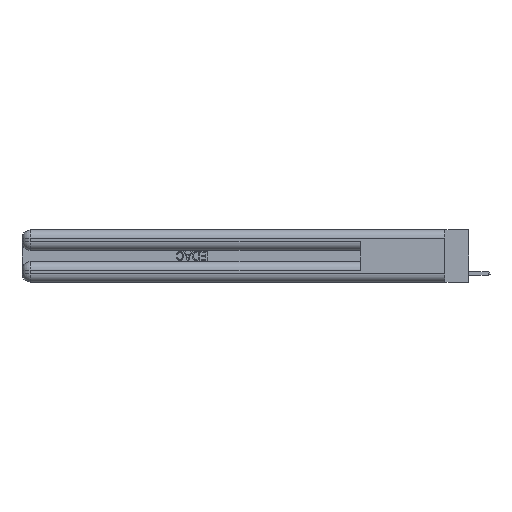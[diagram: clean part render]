
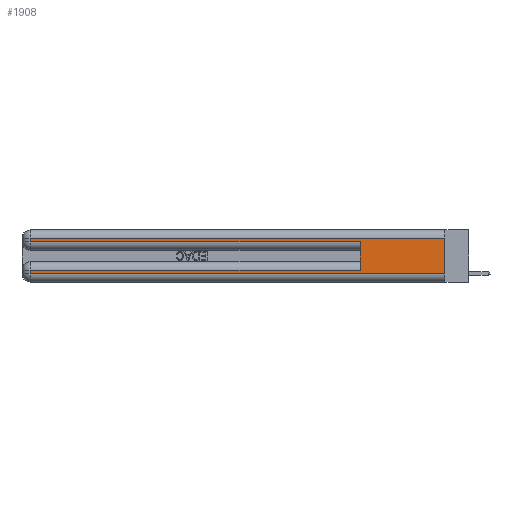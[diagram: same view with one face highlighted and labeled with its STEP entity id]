
A CAD part, left-side view. The second image highlights one B-rep face of the part: STEP entity #1908.
In plain terms, the highlighted planar face has unit normal (-1, 0, 0).
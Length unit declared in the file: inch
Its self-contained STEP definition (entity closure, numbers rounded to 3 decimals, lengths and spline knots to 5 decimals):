
#291 = CARTESIAN_POINT ( 'NONE',  ( 0., 0., 0.37 ) ) ;
#361 = AXIS2_PLACEMENT_3D ( 'NONE', #291, #21021, #10533 ) ;
#381 = CARTESIAN_POINT ( 'NONE',  ( 0., 0.6, 0.085 ) ) ;
#1177 = EDGE_CURVE ( 'NONE', #16755, #10103, #4857, .T. ) ;
#1198 = DIRECTION ( 'NONE',  ( 0., 0., 1. ) ) ;
#1211 = ORIENTED_EDGE ( 'NONE', *, *, #25417, .T. ) ;
#1470 = LINE ( 'NONE', #20380, #2136 ) ;
#1558 = VECTOR ( 'NONE', #1198, 39.37008 ) ;
#1616 = ORIENTED_EDGE ( 'NONE', *, *, #2651, .T. ) ;
#1734 = VECTOR ( 'NONE', #12734, 39.37008 ) ;
#1908 = ADVANCED_FACE ( 'NONE', ( #14744 ), #21427, .F. ) ;
#1928 = VERTEX_POINT ( 'NONE', #25392 ) ;
#2090 = ORIENTED_EDGE ( 'NONE', *, *, #19358, .F. ) ;
#2124 = DIRECTION ( 'NONE',  ( 0., 1., 0. ) ) ;
#2135 = EDGE_CURVE ( 'NONE', #21416, #1928, #24283, .T. ) ;
#2136 = VECTOR ( 'NONE', #7729, 39.37008 ) ;
#2368 = CARTESIAN_POINT ( 'NONE',  ( 0., 2.94, 0.37 ) ) ;
#2477 = VERTEX_POINT ( 'NONE', #16028 ) ;
#2498 = LINE ( 'NONE', #2368, #1734 ) ;
#2587 = VECTOR ( 'NONE', #23390, 39.37008 ) ;
#2651 = EDGE_CURVE ( 'NONE', #9001, #1928, #22695, .T. ) ;
#2717 = ORIENTED_EDGE ( 'NONE', *, *, #9899, .T. ) ;
#3200 = CARTESIAN_POINT ( 'NONE',  ( 0., 0., 0.31 ) ) ;
#3744 = CARTESIAN_POINT ( 'NONE',  ( 0., 0., 0.06 ) ) ;
#4393 = CARTESIAN_POINT ( 'NONE',  ( 0., 2.94, 0.285 ) ) ;
#4735 = EDGE_CURVE ( 'NONE', #26776, #7300, #1470, .T. ) ;
#4857 = LINE ( 'NONE', #15074, #2587 ) ;
#5105 = ORIENTED_EDGE ( 'NONE', *, *, #1177, .T. ) ;
#6921 = VECTOR ( 'NONE', #18528, 39.37008 ) ;
#7300 = VERTEX_POINT ( 'NONE', #13437 ) ;
#7481 = LINE ( 'NONE', #19456, #1558 ) ;
#7729 = DIRECTION ( 'NONE',  ( 0., -1., 0. ) ) ;
#9001 = VERTEX_POINT ( 'NONE', #24707 ) ;
#9186 = VECTOR ( 'NONE', #20363, 39.37008 ) ;
#9899 = EDGE_CURVE ( 'NONE', #21416, #2477, #20532, .T. ) ;
#10103 = VERTEX_POINT ( 'NONE', #21466 ) ;
#10351 = EDGE_LOOP ( 'NONE', ( #10614, #2717, #1211, #20136, #2090, #5105, #12461, #1616 ) ) ;
#10533 = DIRECTION ( 'NONE',  ( 0., 0., -1. ) ) ;
#10614 = ORIENTED_EDGE ( 'NONE', *, *, #2135, .F. ) ;
#11387 = CARTESIAN_POINT ( 'NONE',  ( 0., 2.94, 0.37 ) ) ;
#12461 = ORIENTED_EDGE ( 'NONE', *, *, #12863, .T. ) ;
#12734 = DIRECTION ( 'NONE',  ( 0., 0., -1. ) ) ;
#12863 = EDGE_CURVE ( 'NONE', #10103, #9001, #21742, .T. ) ;
#13144 = VECTOR ( 'NONE', #25565, 39.37008 ) ;
#13437 = CARTESIAN_POINT ( 'NONE',  ( 0., 0.6, 0.285 ) ) ;
#14744 = FACE_OUTER_BOUND ( 'NONE', #10351, .T. ) ;
#15074 = CARTESIAN_POINT ( 'NONE',  ( 0., 0., 0.085 ) ) ;
#16028 = CARTESIAN_POINT ( 'NONE',  ( 0., 2.94, 0.31 ) ) ;
#16755 = VERTEX_POINT ( 'NONE', #381 ) ;
#18528 = DIRECTION ( 'NONE',  ( 0., 0., -1. ) ) ;
#19358 = EDGE_CURVE ( 'NONE', #16755, #7300, #7481, .T. ) ;
#19456 = CARTESIAN_POINT ( 'NONE',  ( 0., 0.6, 0.145 ) ) ;
#20120 = VECTOR ( 'NONE', #2124, 39.37008 ) ;
#20136 = ORIENTED_EDGE ( 'NONE', *, *, #4735, .T. ) ;
#20363 = DIRECTION ( 'NONE',  ( 0., -1., 0. ) ) ;
#20380 = CARTESIAN_POINT ( 'NONE',  ( 0., 0., 0.285 ) ) ;
#20430 = CARTESIAN_POINT ( 'NONE',  ( 0., 0., 0.37 ) ) ;
#20532 = LINE ( 'NONE', #22461, #20120 ) ;
#21021 = DIRECTION ( 'NONE',  ( 1., 0., 0. ) ) ;
#21416 = VERTEX_POINT ( 'NONE', #3200 ) ;
#21427 = PLANE ( 'NONE',  #361 ) ;
#21466 = CARTESIAN_POINT ( 'NONE',  ( 0., 2.94, 0.085 ) ) ;
#21742 = LINE ( 'NONE', #11387, #13144 ) ;
#22461 = CARTESIAN_POINT ( 'NONE',  ( 0., 0., 0.31 ) ) ;
#22695 = LINE ( 'NONE', #3744, #9186 ) ;
#23390 = DIRECTION ( 'NONE',  ( 0., 1., 0. ) ) ;
#24283 = LINE ( 'NONE', #20430, #6921 ) ;
#24707 = CARTESIAN_POINT ( 'NONE',  ( 0., 2.94, 0.06 ) ) ;
#25392 = CARTESIAN_POINT ( 'NONE',  ( 0., 0., 0.06 ) ) ;
#25417 = EDGE_CURVE ( 'NONE', #2477, #26776, #2498, .T. ) ;
#25565 = DIRECTION ( 'NONE',  ( 0., 0., -1. ) ) ;
#26776 = VERTEX_POINT ( 'NONE', #4393 ) ;
